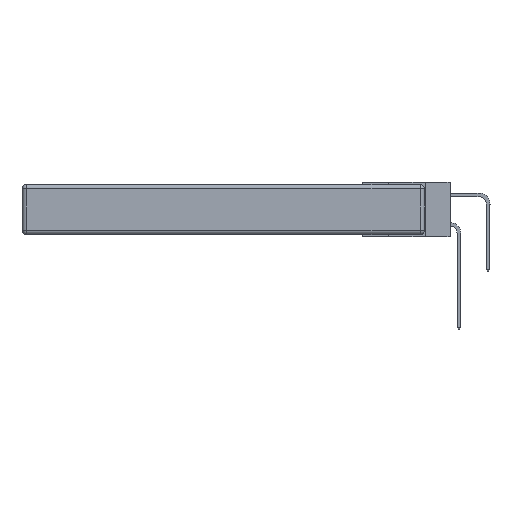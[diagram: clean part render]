
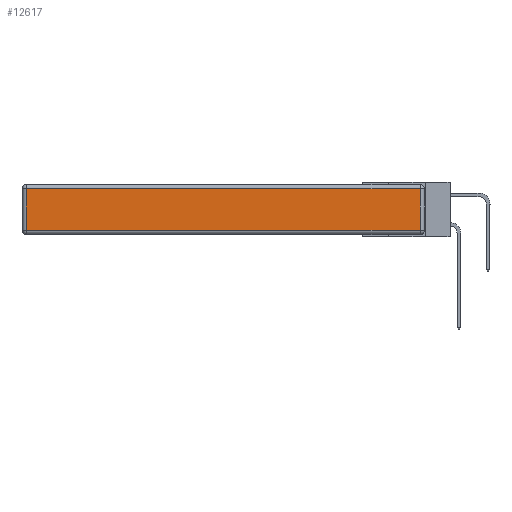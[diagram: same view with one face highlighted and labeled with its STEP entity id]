
A CAD part, left-side view. The second image highlights one B-rep face of the part: STEP entity #12617.
In plain terms, the highlighted planar face has unit normal (-1, 0, 0).
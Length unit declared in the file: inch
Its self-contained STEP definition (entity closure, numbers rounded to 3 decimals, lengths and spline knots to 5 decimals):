
#1218 = EDGE_CURVE ( 'NONE', #3263, #16253, #11678, .T. ) ;
#1305 = DIRECTION ( 'NONE',  ( -1., 0., 0. ) ) ;
#1442 = CARTESIAN_POINT ( 'NONE',  ( 0., 2.72, -0.343 ) ) ;
#1448 = VERTEX_POINT ( 'NONE', #13050 ) ;
#1475 = EDGE_CURVE ( 'NONE', #16253, #1448, #14717, .T. ) ;
#1586 = DIRECTION ( 'NONE',  ( 0., -1., 0. ) ) ;
#2420 = VECTOR ( 'NONE', #3622, 39.37008 ) ;
#2537 = EDGE_CURVE ( 'NONE', #1448, #8554, #16834, .T. ) ;
#3028 = CARTESIAN_POINT ( 'NONE',  ( 0., 0., -0.313 ) ) ;
#3089 = VECTOR ( 'NONE', #3952, 39.37008 ) ;
#3263 = VERTEX_POINT ( 'NONE', #8383 ) ;
#3622 = DIRECTION ( 'NONE',  ( 0., 0., 1. ) ) ;
#3952 = DIRECTION ( 'NONE',  ( 0., 0., -1. ) ) ;
#4802 = DIRECTION ( 'NONE',  ( 0., 1., 0. ) ) ;
#6691 = ORIENTED_EDGE ( 'NONE', *, *, #15871, .T. ) ;
#7618 = VECTOR ( 'NONE', #4802, 39.37008 ) ;
#8383 = CARTESIAN_POINT ( 'NONE',  ( 0., 0.03, -0.313 ) ) ;
#8554 = VERTEX_POINT ( 'NONE', #13808 ) ;
#9203 = EDGE_LOOP ( 'NONE', ( #6691, #11710, #17833, #16247 ) ) ;
#9707 = CARTESIAN_POINT ( 'NONE',  ( 0., 0., -0.343 ) ) ;
#11498 = CARTESIAN_POINT ( 'NONE',  ( 0., 2.75, -0.03 ) ) ;
#11678 = LINE ( 'NONE', #14518, #2420 ) ;
#11710 = ORIENTED_EDGE ( 'NONE', *, *, #1218, .T. ) ;
#12351 = PLANE ( 'NONE',  #16415 ) ;
#12617 = ADVANCED_FACE ( 'NONE', ( #14346 ), #12351, .T. ) ;
#12798 = VECTOR ( 'NONE', #1586, 39.37008 ) ;
#12940 = CARTESIAN_POINT ( 'NONE',  ( 0., 0.03, -0.03 ) ) ;
#13050 = CARTESIAN_POINT ( 'NONE',  ( 0., 2.72, -0.03 ) ) ;
#13808 = CARTESIAN_POINT ( 'NONE',  ( 0., 2.72, -0.313 ) ) ;
#14346 = FACE_OUTER_BOUND ( 'NONE', #9203, .T. ) ;
#14518 = CARTESIAN_POINT ( 'NONE',  ( 0., 0.03, -0.343 ) ) ;
#14717 = LINE ( 'NONE', #11498, #7618 ) ;
#15364 = DIRECTION ( 'NONE',  ( 0., 0., 1. ) ) ;
#15871 = EDGE_CURVE ( 'NONE', #8554, #3263, #17747, .T. ) ;
#16247 = ORIENTED_EDGE ( 'NONE', *, *, #2537, .T. ) ;
#16253 = VERTEX_POINT ( 'NONE', #12940 ) ;
#16415 = AXIS2_PLACEMENT_3D ( 'NONE', #9707, #1305, #15364 ) ;
#16834 = LINE ( 'NONE', #1442, #3089 ) ;
#17747 = LINE ( 'NONE', #3028, #12798 ) ;
#17833 = ORIENTED_EDGE ( 'NONE', *, *, #1475, .T. ) ;
